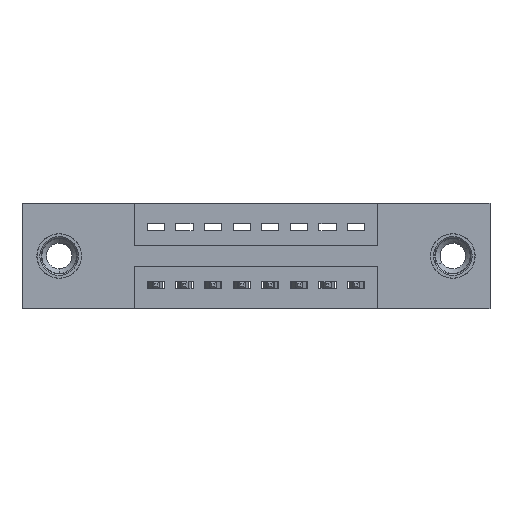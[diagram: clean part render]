
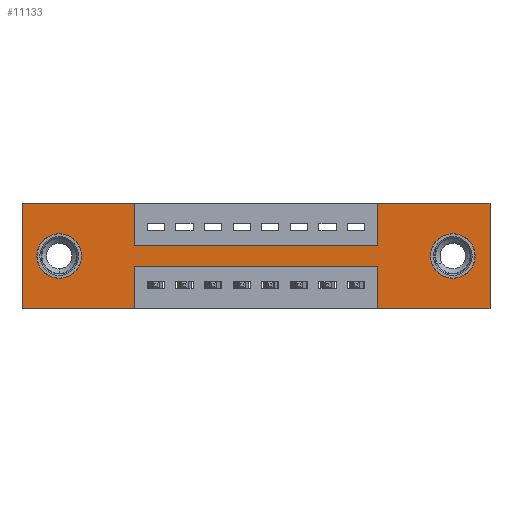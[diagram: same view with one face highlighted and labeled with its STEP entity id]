
A CAD part, front view. The second image highlights one B-rep face of the part: STEP entity #11133.
In plain terms, the highlighted planar face has unit normal (0, -1, 0).
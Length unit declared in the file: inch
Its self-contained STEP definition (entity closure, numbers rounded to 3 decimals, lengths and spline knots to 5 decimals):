
#76 = VERTEX_POINT ( 'NONE', #10153 ) ;
#98 = EDGE_LOOP ( 'NONE', ( #3852, #1758 ) ) ;
#204 = VERTEX_POINT ( 'NONE', #7653 ) ;
#246 = CIRCLE ( 'NONE', #4041, 0.078 ) ;
#271 = DIRECTION ( 'NONE',  ( 0., 0., -1. ) ) ;
#332 = CARTESIAN_POINT ( 'NONE',  ( 1.2425, 0., -0.37 ) ) ;
#337 = DIRECTION ( 'NONE',  ( 0., 0., -1. ) ) ;
#371 = LINE ( 'NONE', #332, #3210 ) ;
#402 = LINE ( 'NONE', #10810, #970 ) ;
#419 = DIRECTION ( 'NONE',  ( 0., 0., 1. ) ) ;
#645 = EDGE_CURVE ( 'NONE', #10321, #8718, #2614, .T. ) ;
#778 = DIRECTION ( 'NONE',  ( 0., 0., 1. ) ) ;
#875 = EDGE_CURVE ( 'NONE', #10750, #76, #7728, .T. ) ;
#970 = VECTOR ( 'NONE', #11799, 39.37008 ) ;
#1051 = CARTESIAN_POINT ( 'NONE',  ( 0.3925, 0., -0.15 ) ) ;
#1096 = LINE ( 'NONE', #4539, #1979 ) ;
#1135 = VECTOR ( 'NONE', #9630, 39.37008 ) ;
#1328 = FACE_BOUND ( 'NONE', #4933, .T. ) ;
#1337 = CARTESIAN_POINT ( 'NONE',  ( 1.2425, 0., -0.37 ) ) ;
#1722 = AXIS2_PLACEMENT_3D ( 'NONE', #3115, #10289, #419 ) ;
#1758 = ORIENTED_EDGE ( 'NONE', *, *, #11252, .T. ) ;
#1777 = DIRECTION ( 'NONE',  ( 0., 0., -1. ) ) ;
#1979 = VECTOR ( 'NONE', #7311, 39.37008 ) ;
#2134 = LINE ( 'NONE', #3049, #4111 ) ;
#2233 = LINE ( 'NONE', #4417, #10639 ) ;
#2398 = ORIENTED_EDGE ( 'NONE', *, *, #11575, .F. ) ;
#2614 = LINE ( 'NONE', #3625, #7438 ) ;
#3049 = CARTESIAN_POINT ( 'NONE',  ( 0.3925, 0., 0. ) ) ;
#3110 = EDGE_CURVE ( 'NONE', #204, #8295, #402, .T. ) ;
#3115 = CARTESIAN_POINT ( 'NONE',  ( 0.13, 0., -0.185 ) ) ;
#3128 = LINE ( 'NONE', #11599, #8423 ) ;
#3210 = VECTOR ( 'NONE', #10449, 39.37008 ) ;
#3333 = FACE_BOUND ( 'NONE', #98, .T. ) ;
#3432 = ORIENTED_EDGE ( 'NONE', *, *, #10231, .F. ) ;
#3487 = EDGE_CURVE ( 'NONE', #9289, #4151, #246, .T. ) ;
#3512 = ORIENTED_EDGE ( 'NONE', *, *, #6559, .F. ) ;
#3625 = CARTESIAN_POINT ( 'NONE',  ( 1.635, 0., 0. ) ) ;
#3841 = LINE ( 'NONE', #7858, #1135 ) ;
#3852 = ORIENTED_EDGE ( 'NONE', *, *, #5473, .T. ) ;
#3889 = ORIENTED_EDGE ( 'NONE', *, *, #3110, .F. ) ;
#4041 = AXIS2_PLACEMENT_3D ( 'NONE', #5552, #8279, #4793 ) ;
#4111 = VECTOR ( 'NONE', #271, 39.37008 ) ;
#4138 = CARTESIAN_POINT ( 'NONE',  ( 0., 0., 0. ) ) ;
#4144 = CARTESIAN_POINT ( 'NONE',  ( 1.505, 0., -0.185 ) ) ;
#4151 = VERTEX_POINT ( 'NONE', #6066 ) ;
#4417 = CARTESIAN_POINT ( 'NONE',  ( 0., 0., 0. ) ) ;
#4443 = EDGE_CURVE ( 'NONE', #5857, #9338, #2233, .T. ) ;
#4458 = EDGE_CURVE ( 'NONE', #76, #9384, #5075, .T. ) ;
#4492 = DIRECTION ( 'NONE',  ( 0., 0., 1. ) ) ;
#4539 = CARTESIAN_POINT ( 'NONE',  ( 0., 0., -0.37 ) ) ;
#4648 = CARTESIAN_POINT ( 'NONE',  ( 1.505, 0., -0.107 ) ) ;
#4793 = DIRECTION ( 'NONE',  ( 0., 0., 1. ) ) ;
#4875 = DIRECTION ( 'NONE',  ( 0., 1., 0. ) ) ;
#4932 = DIRECTION ( 'NONE',  ( 0., 1., 0. ) ) ;
#4933 = EDGE_LOOP ( 'NONE', ( #11735, #6773 ) ) ;
#5004 = CARTESIAN_POINT ( 'NONE',  ( 0., 0., -0.37 ) ) ;
#5011 = VECTOR ( 'NONE', #8387, 39.37008 ) ;
#5075 = LINE ( 'NONE', #7185, #8784 ) ;
#5473 = EDGE_CURVE ( 'NONE', #9090, #6109, #11516, .T. ) ;
#5525 = EDGE_CURVE ( 'NONE', #9338, #7133, #3128, .T. ) ;
#5552 = CARTESIAN_POINT ( 'NONE',  ( 0.13, 0., -0.185 ) ) ;
#5841 = CARTESIAN_POINT ( 'NONE',  ( 1.635, 0., 0. ) ) ;
#5857 = VERTEX_POINT ( 'NONE', #5004 ) ;
#5974 = VERTEX_POINT ( 'NONE', #1337 ) ;
#6049 = AXIS2_PLACEMENT_3D ( 'NONE', #4144, #4932, #10343 ) ;
#6066 = CARTESIAN_POINT ( 'NONE',  ( 0.13, 0., -0.263 ) ) ;
#6098 = ORIENTED_EDGE ( 'NONE', *, *, #7991, .F. ) ;
#6109 = VERTEX_POINT ( 'NONE', #8752 ) ;
#6496 = ORIENTED_EDGE ( 'NONE', *, *, #10835, .F. ) ;
#6559 = EDGE_CURVE ( 'NONE', #7133, #10750, #2134, .T. ) ;
#6573 = DIRECTION ( 'NONE',  ( 0., 0., -1. ) ) ;
#6674 = VERTEX_POINT ( 'NONE', #7723 ) ;
#6690 = ORIENTED_EDGE ( 'NONE', *, *, #9392, .F. ) ;
#6763 = CARTESIAN_POINT ( 'NONE',  ( 1.2425, 0., 0. ) ) ;
#6773 = ORIENTED_EDGE ( 'NONE', *, *, #9753, .T. ) ;
#6849 = EDGE_LOOP ( 'NONE', ( #3889, #6496, #6098, #2398, #9317, #6690, #11059, #9930, #3512, #9534, #9427, #3432 ) ) ;
#7133 = VERTEX_POINT ( 'NONE', #9676 ) ;
#7185 = CARTESIAN_POINT ( 'NONE',  ( 1.2425, 0., 0. ) ) ;
#7214 = CARTESIAN_POINT ( 'NONE',  ( 0.3925, 0., -0.37 ) ) ;
#7311 = DIRECTION ( 'NONE',  ( -1., 0., 0. ) ) ;
#7438 = VECTOR ( 'NONE', #1777, 39.37008 ) ;
#7653 = CARTESIAN_POINT ( 'NONE',  ( 0.3925, 0., -0.22 ) ) ;
#7689 = CARTESIAN_POINT ( 'NONE',  ( 0.3925, 0., -0.15 ) ) ;
#7723 = CARTESIAN_POINT ( 'NONE',  ( 1.2425, 0., -0.22 ) ) ;
#7728 = LINE ( 'NONE', #1051, #5011 ) ;
#7732 = CARTESIAN_POINT ( 'NONE',  ( 1.635, 0., -0.37 ) ) ;
#7858 = CARTESIAN_POINT ( 'NONE',  ( 0.3925, 0., -0.22 ) ) ;
#7882 = CARTESIAN_POINT ( 'NONE',  ( 0., 0., 0. ) ) ;
#7899 = DIRECTION ( 'NONE',  ( 1., 0., 0. ) ) ;
#7991 = EDGE_CURVE ( 'NONE', #5974, #6674, #371, .T. ) ;
#8279 = DIRECTION ( 'NONE',  ( 0., 1., 0. ) ) ;
#8289 = AXIS2_PLACEMENT_3D ( 'NONE', #10327, #4875, #337 ) ;
#8295 = VERTEX_POINT ( 'NONE', #7214 ) ;
#8320 = VECTOR ( 'NONE', #9649, 39.37008 ) ;
#8387 = DIRECTION ( 'NONE',  ( 1., 0., 0. ) ) ;
#8423 = VECTOR ( 'NONE', #7899, 39.37008 ) ;
#8523 = CIRCLE ( 'NONE', #6049, 0.078 ) ;
#8717 = CARTESIAN_POINT ( 'NONE',  ( 0.13, 0., -0.107 ) ) ;
#8718 = VERTEX_POINT ( 'NONE', #7732 ) ;
#8752 = CARTESIAN_POINT ( 'NONE',  ( 1.505, 0., -0.263 ) ) ;
#8784 = VECTOR ( 'NONE', #4492, 39.37008 ) ;
#8884 = FACE_OUTER_BOUND ( 'NONE', #6849, .T. ) ;
#9090 = VERTEX_POINT ( 'NONE', #4648 ) ;
#9239 = CARTESIAN_POINT ( 'NONE',  ( 0., 0., -0.37 ) ) ;
#9271 = DIRECTION ( 'NONE',  ( 0., -1., 0. ) ) ;
#9289 = VERTEX_POINT ( 'NONE', #8717 ) ;
#9314 = DIRECTION ( 'NONE',  ( -1., 0., 0. ) ) ;
#9317 = ORIENTED_EDGE ( 'NONE', *, *, #645, .F. ) ;
#9338 = VERTEX_POINT ( 'NONE', #7882 ) ;
#9384 = VERTEX_POINT ( 'NONE', #6763 ) ;
#9392 = EDGE_CURVE ( 'NONE', #9384, #10321, #10741, .T. ) ;
#9427 = ORIENTED_EDGE ( 'NONE', *, *, #4443, .F. ) ;
#9534 = ORIENTED_EDGE ( 'NONE', *, *, #5525, .F. ) ;
#9630 = DIRECTION ( 'NONE',  ( -1., 0., 0. ) ) ;
#9649 = DIRECTION ( 'NONE',  ( 1., 0., 0. ) ) ;
#9676 = CARTESIAN_POINT ( 'NONE',  ( 0.3925, 0., 0. ) ) ;
#9753 = EDGE_CURVE ( 'NONE', #4151, #9289, #10282, .T. ) ;
#9930 = ORIENTED_EDGE ( 'NONE', *, *, #875, .F. ) ;
#10141 = PLANE ( 'NONE',  #10174 ) ;
#10153 = CARTESIAN_POINT ( 'NONE',  ( 1.2425, 0., -0.15 ) ) ;
#10174 = AXIS2_PLACEMENT_3D ( 'NONE', #11158, #9271, #6573 ) ;
#10231 = EDGE_CURVE ( 'NONE', #8295, #5857, #10429, .T. ) ;
#10282 = CIRCLE ( 'NONE', #1722, 0.078 ) ;
#10289 = DIRECTION ( 'NONE',  ( 0., 1., 0. ) ) ;
#10321 = VERTEX_POINT ( 'NONE', #5841 ) ;
#10327 = CARTESIAN_POINT ( 'NONE',  ( 1.505, 0., -0.185 ) ) ;
#10343 = DIRECTION ( 'NONE',  ( 0., 0., -1. ) ) ;
#10429 = LINE ( 'NONE', #9239, #11144 ) ;
#10449 = DIRECTION ( 'NONE',  ( 0., 0., 1. ) ) ;
#10639 = VECTOR ( 'NONE', #778, 39.37008 ) ;
#10741 = LINE ( 'NONE', #4138, #8320 ) ;
#10750 = VERTEX_POINT ( 'NONE', #7689 ) ;
#10810 = CARTESIAN_POINT ( 'NONE',  ( 0.3925, 0., -0.37 ) ) ;
#10835 = EDGE_CURVE ( 'NONE', #6674, #204, #3841, .T. ) ;
#11059 = ORIENTED_EDGE ( 'NONE', *, *, #4458, .F. ) ;
#11133 = ADVANCED_FACE ( 'NONE', ( #3333, #1328, #8884 ), #10141, .T. ) ;
#11144 = VECTOR ( 'NONE', #9314, 39.37008 ) ;
#11158 = CARTESIAN_POINT ( 'NONE',  ( 0., 0., -0.37 ) ) ;
#11252 = EDGE_CURVE ( 'NONE', #6109, #9090, #8523, .T. ) ;
#11516 = CIRCLE ( 'NONE', #8289, 0.078 ) ;
#11575 = EDGE_CURVE ( 'NONE', #8718, #5974, #1096, .T. ) ;
#11599 = CARTESIAN_POINT ( 'NONE',  ( 0., 0., 0. ) ) ;
#11735 = ORIENTED_EDGE ( 'NONE', *, *, #3487, .T. ) ;
#11799 = DIRECTION ( 'NONE',  ( 0., 0., -1. ) ) ;
